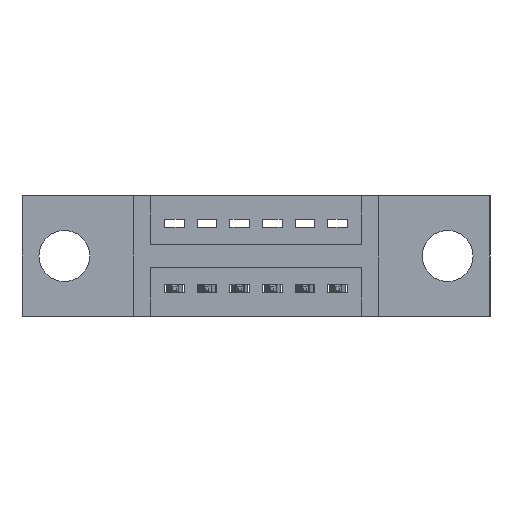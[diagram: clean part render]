
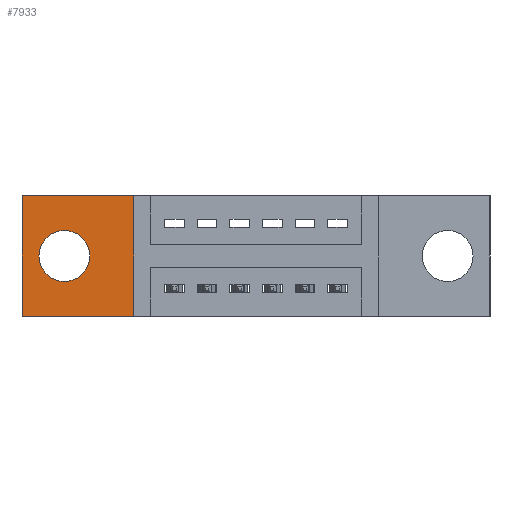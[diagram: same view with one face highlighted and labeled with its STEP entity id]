
A CAD part, front view. The second image highlights one B-rep face of the part: STEP entity #7933.
In plain terms, the highlighted planar face has unit normal (0, -1, 0).
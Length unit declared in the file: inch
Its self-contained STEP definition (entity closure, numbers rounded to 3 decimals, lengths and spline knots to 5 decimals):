
#46 = CARTESIAN_POINT ( 'NONE',  ( 0., 0.11, -0.37 ) ) ;
#66 = LINE ( 'NONE', #7088, #9130 ) ;
#329 = DIRECTION ( 'NONE',  ( 0., -1., 0. ) ) ;
#356 = CARTESIAN_POINT ( 'NONE',  ( 0., 0.11, -0.37 ) ) ;
#380 = VERTEX_POINT ( 'NONE', #46 ) ;
#612 = FACE_BOUND ( 'NONE', #5652, .T. ) ;
#614 = DIRECTION ( 'NONE',  ( 0., 0., -1. ) ) ;
#626 = EDGE_CURVE ( 'NONE', #2508, #5419, #2586, .T. ) ;
#750 = ORIENTED_EDGE ( 'NONE', *, *, #4584, .F. ) ;
#787 = VERTEX_POINT ( 'NONE', #4835 ) ;
#869 = CARTESIAN_POINT ( 'NONE',  ( 0.3425, 0.11, -0.37 ) ) ;
#995 = ORIENTED_EDGE ( 'NONE', *, *, #6317, .T. ) ;
#1204 = DIRECTION ( 'NONE',  ( 0., 0., -1. ) ) ;
#1630 = EDGE_CURVE ( 'NONE', #5029, #5360, #2339, .T. ) ;
#2339 = CIRCLE ( 'NONE', #8433, 0.078 ) ;
#2508 = VERTEX_POINT ( 'NONE', #869 ) ;
#2515 = ORIENTED_EDGE ( 'NONE', *, *, #626, .T. ) ;
#2586 = LINE ( 'NONE', #7584, #9433 ) ;
#2641 = CARTESIAN_POINT ( 'NONE',  ( 0.13, 0.11, -0.185 ) ) ;
#2663 = DIRECTION ( 'NONE',  ( -1., 0., 0. ) ) ;
#3286 = FACE_OUTER_BOUND ( 'NONE', #5205, .T. ) ;
#4466 = VECTOR ( 'NONE', #8227, 39.37008 ) ;
#4571 = CARTESIAN_POINT ( 'NONE',  ( 0.13, 0.11, -0.185 ) ) ;
#4584 = EDGE_CURVE ( 'NONE', #5360, #5029, #5047, .T. ) ;
#4669 = LINE ( 'NONE', #6574, #6379 ) ;
#4696 = DIRECTION ( 'NONE',  ( 0., 0., 1. ) ) ;
#4835 = CARTESIAN_POINT ( 'NONE',  ( 0., 0.11, 0. ) ) ;
#4946 = DIRECTION ( 'NONE',  ( 0., -1., 0. ) ) ;
#5029 = VERTEX_POINT ( 'NONE', #8643 ) ;
#5047 = CIRCLE ( 'NONE', #7226, 0.078 ) ;
#5172 = LINE ( 'NONE', #6116, #4466 ) ;
#5205 = EDGE_LOOP ( 'NONE', ( #5459, #8287, #2515, #995 ) ) ;
#5360 = VERTEX_POINT ( 'NONE', #6833 ) ;
#5419 = VERTEX_POINT ( 'NONE', #6534 ) ;
#5459 = ORIENTED_EDGE ( 'NONE', *, *, #7482, .T. ) ;
#5652 = EDGE_LOOP ( 'NONE', ( #750, #6598 ) ) ;
#6116 = CARTESIAN_POINT ( 'NONE',  ( 0., 0.11, -0.37 ) ) ;
#6317 = EDGE_CURVE ( 'NONE', #5419, #787, #66, .T. ) ;
#6319 = AXIS2_PLACEMENT_3D ( 'NONE', #356, #4946, #8583 ) ;
#6379 = VECTOR ( 'NONE', #614, 39.37008 ) ;
#6534 = CARTESIAN_POINT ( 'NONE',  ( 0.3425, 0.11, 0. ) ) ;
#6574 = CARTESIAN_POINT ( 'NONE',  ( 0., 0.11, 0. ) ) ;
#6598 = ORIENTED_EDGE ( 'NONE', *, *, #1630, .F. ) ;
#6833 = CARTESIAN_POINT ( 'NONE',  ( 0.13, 0.11, -0.107 ) ) ;
#7035 = PLANE ( 'NONE',  #6319 ) ;
#7088 = CARTESIAN_POINT ( 'NONE',  ( 0., 0.11, 0. ) ) ;
#7226 = AXIS2_PLACEMENT_3D ( 'NONE', #2641, #7763, #1204 ) ;
#7482 = EDGE_CURVE ( 'NONE', #787, #380, #4669, .T. ) ;
#7584 = CARTESIAN_POINT ( 'NONE',  ( 0.3425, 0.11, 0. ) ) ;
#7763 = DIRECTION ( 'NONE',  ( 0., -1., 0. ) ) ;
#7784 = DIRECTION ( 'NONE',  ( 0., 0., -1. ) ) ;
#7933 = ADVANCED_FACE ( 'NONE', ( #612, #3286 ), #7035, .T. ) ;
#8227 = DIRECTION ( 'NONE',  ( 1., 0., 0. ) ) ;
#8287 = ORIENTED_EDGE ( 'NONE', *, *, #9364, .T. ) ;
#8433 = AXIS2_PLACEMENT_3D ( 'NONE', #4571, #329, #7784 ) ;
#8583 = DIRECTION ( 'NONE',  ( 0., 0., -1. ) ) ;
#8643 = CARTESIAN_POINT ( 'NONE',  ( 0.13, 0.11, -0.263 ) ) ;
#9130 = VECTOR ( 'NONE', #2663, 39.37008 ) ;
#9364 = EDGE_CURVE ( 'NONE', #380, #2508, #5172, .T. ) ;
#9433 = VECTOR ( 'NONE', #4696, 39.37008 ) ;
